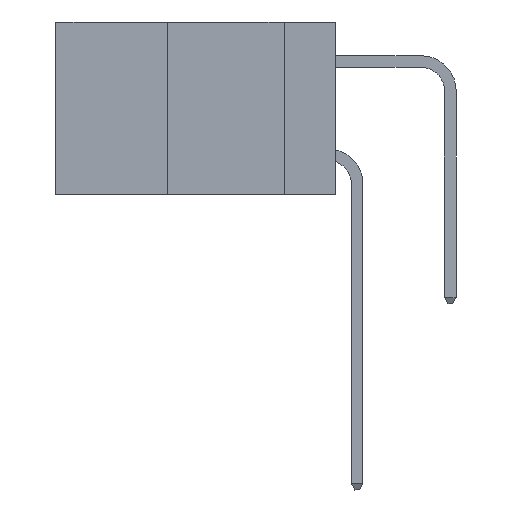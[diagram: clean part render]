
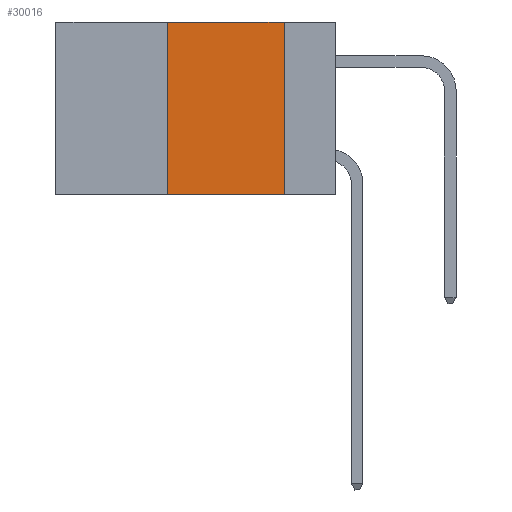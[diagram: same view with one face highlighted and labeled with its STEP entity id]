
A CAD part, left-side view. The second image highlights one B-rep face of the part: STEP entity #30016.
In plain terms, the highlighted planar face has unit normal (-1, 0, 0).
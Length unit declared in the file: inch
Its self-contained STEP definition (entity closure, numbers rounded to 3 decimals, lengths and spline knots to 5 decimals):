
#254 = CARTESIAN_POINT ( 'NONE',  ( 0., 0.11, 0. ) ) ;
#318 = EDGE_CURVE ( 'NONE', #11437, #25399, #3220, .T. ) ;
#537 = CARTESIAN_POINT ( 'NONE',  ( 0., 0.6, -0.37 ) ) ;
#1148 = LINE ( 'NONE', #13758, #3673 ) ;
#2919 = DIRECTION ( 'NONE',  ( 0., -1., 0. ) ) ;
#3220 = LINE ( 'NONE', #31678, #13212 ) ;
#3673 = VECTOR ( 'NONE', #2919, 39.37008 ) ;
#3677 = CARTESIAN_POINT ( 'NONE',  ( 0., 0.36, 0. ) ) ;
#7398 = VERTEX_POINT ( 'NONE', #13847 ) ;
#9042 = DIRECTION ( 'NONE',  ( 0., 0., 1. ) ) ;
#11437 = VERTEX_POINT ( 'NONE', #254 ) ;
#12028 = LINE ( 'NONE', #3677, #28760 ) ;
#13212 = VECTOR ( 'NONE', #18355, 39.37008 ) ;
#13758 = CARTESIAN_POINT ( 'NONE',  ( 0., 0.6, 0. ) ) ;
#13847 = CARTESIAN_POINT ( 'NONE',  ( 0., 0.36, 0. ) ) ;
#14941 = CARTESIAN_POINT ( 'NONE',  ( 0., 0.6, 0. ) ) ;
#15455 = ORIENTED_EDGE ( 'NONE', *, *, #32226, .T. ) ;
#17196 = DIRECTION ( 'NONE',  ( 1., 0., 0. ) ) ;
#18130 = FACE_OUTER_BOUND ( 'NONE', #32039, .T. ) ;
#18191 = CARTESIAN_POINT ( 'NONE',  ( 0., 0.11, -0.37 ) ) ;
#18355 = DIRECTION ( 'NONE',  ( 0., 0., -1. ) ) ;
#19840 = EDGE_CURVE ( 'NONE', #33614, #7398, #12028, .T. ) ;
#20059 = VECTOR ( 'NONE', #21913, 39.37008 ) ;
#20291 = EDGE_CURVE ( 'NONE', #7398, #11437, #1148, .T. ) ;
#20315 = PLANE ( 'NONE',  #26105 ) ;
#21913 = DIRECTION ( 'NONE',  ( 0., -1., 0. ) ) ;
#22556 = DIRECTION ( 'NONE',  ( 0., 0., -1. ) ) ;
#22564 = LINE ( 'NONE', #537, #20059 ) ;
#25399 = VERTEX_POINT ( 'NONE', #18191 ) ;
#26105 = AXIS2_PLACEMENT_3D ( 'NONE', #14941, #17196, #22556 ) ;
#27160 = ORIENTED_EDGE ( 'NONE', *, *, #20291, .F. ) ;
#28760 = VECTOR ( 'NONE', #9042, 39.37008 ) ;
#29061 = ORIENTED_EDGE ( 'NONE', *, *, #19840, .F. ) ;
#30016 = ADVANCED_FACE ( 'NONE', ( #18130 ), #20315, .F. ) ;
#30593 = ORIENTED_EDGE ( 'NONE', *, *, #318, .F. ) ;
#31678 = CARTESIAN_POINT ( 'NONE',  ( 0., 0.11, 0. ) ) ;
#32039 = EDGE_LOOP ( 'NONE', ( #30593, #27160, #29061, #15455 ) ) ;
#32088 = CARTESIAN_POINT ( 'NONE',  ( 0., 0.36, -0.37 ) ) ;
#32226 = EDGE_CURVE ( 'NONE', #33614, #25399, #22564, .T. ) ;
#33614 = VERTEX_POINT ( 'NONE', #32088 ) ;
